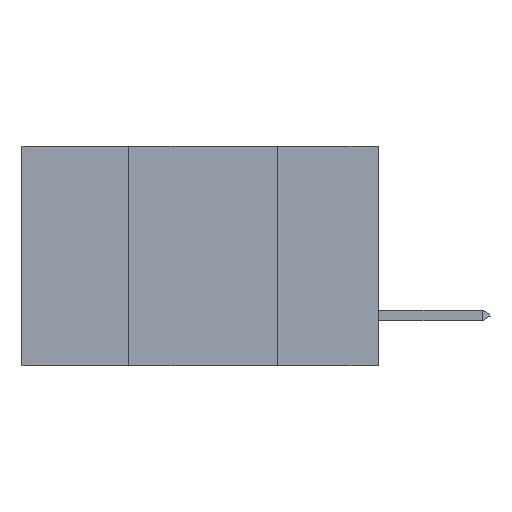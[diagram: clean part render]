
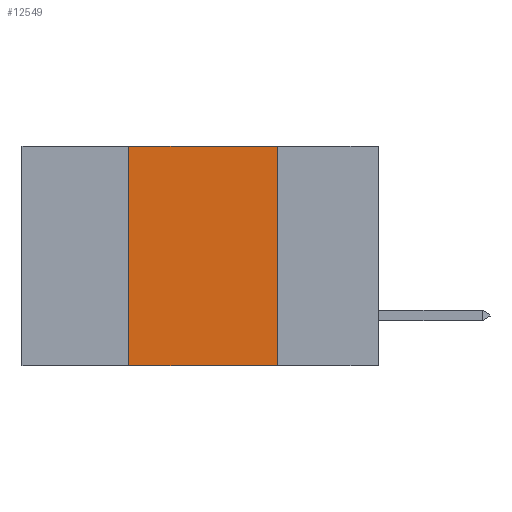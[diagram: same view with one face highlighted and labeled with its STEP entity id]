
A CAD part, left-side view. The second image highlights one B-rep face of the part: STEP entity #12549.
In plain terms, the highlighted planar face has unit normal (-1, 0, 0).
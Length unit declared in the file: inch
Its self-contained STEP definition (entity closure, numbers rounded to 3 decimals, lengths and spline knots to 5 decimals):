
#372 = LINE ( 'NONE', #12339, #6073 ) ;
#637 = EDGE_CURVE ( 'NONE', #7337, #4978, #2503, .T. ) ;
#995 = EDGE_CURVE ( 'NONE', #4978, #8960, #372, .T. ) ;
#1590 = LINE ( 'NONE', #6500, #5011 ) ;
#1611 = CARTESIAN_POINT ( 'NONE',  ( 0., 0.6, 0. ) ) ;
#1785 = DIRECTION ( 'NONE',  ( 0., 0., -1. ) ) ;
#2177 = VERTEX_POINT ( 'NONE', #12095 ) ;
#2503 = LINE ( 'NONE', #1611, #7447 ) ;
#2643 = CARTESIAN_POINT ( 'NONE',  ( 0., 0.6, -0.37 ) ) ;
#2696 = DIRECTION ( 'NONE',  ( 0., -1., 0. ) ) ;
#2707 = VECTOR ( 'NONE', #7983, 39.37008 ) ;
#3459 = EDGE_LOOP ( 'NONE', ( #6336, #8655, #12703, #9341 ) ) ;
#4978 = VERTEX_POINT ( 'NONE', #8935 ) ;
#5011 = VECTOR ( 'NONE', #10710, 39.37008 ) ;
#5422 = EDGE_CURVE ( 'NONE', #2177, #8960, #8772, .T. ) ;
#6073 = VECTOR ( 'NONE', #1785, 39.37008 ) ;
#6336 = ORIENTED_EDGE ( 'NONE', *, *, #995, .F. ) ;
#6500 = CARTESIAN_POINT ( 'NONE',  ( 0., 0.42, 0. ) ) ;
#7302 = DIRECTION ( 'NONE',  ( 1., 0., 0. ) ) ;
#7337 = VERTEX_POINT ( 'NONE', #11039 ) ;
#7447 = VECTOR ( 'NONE', #2696, 39.37008 ) ;
#7983 = DIRECTION ( 'NONE',  ( 0., -1., 0. ) ) ;
#8436 = DIRECTION ( 'NONE',  ( 0., 0., -1. ) ) ;
#8479 = CARTESIAN_POINT ( 'NONE',  ( 0., 0.6, 0. ) ) ;
#8655 = ORIENTED_EDGE ( 'NONE', *, *, #637, .F. ) ;
#8772 = LINE ( 'NONE', #2643, #2707 ) ;
#8935 = CARTESIAN_POINT ( 'NONE',  ( 0., 0.17, 0. ) ) ;
#8960 = VERTEX_POINT ( 'NONE', #12681 ) ;
#9333 = PLANE ( 'NONE',  #11163 ) ;
#9341 = ORIENTED_EDGE ( 'NONE', *, *, #5422, .T. ) ;
#10710 = DIRECTION ( 'NONE',  ( 0., 0., 1. ) ) ;
#11039 = CARTESIAN_POINT ( 'NONE',  ( 0., 0.42, 0. ) ) ;
#11163 = AXIS2_PLACEMENT_3D ( 'NONE', #8479, #7302, #8436 ) ;
#11909 = EDGE_CURVE ( 'NONE', #2177, #7337, #1590, .T. ) ;
#11938 = FACE_OUTER_BOUND ( 'NONE', #3459, .T. ) ;
#12095 = CARTESIAN_POINT ( 'NONE',  ( 0., 0.42, -0.37 ) ) ;
#12339 = CARTESIAN_POINT ( 'NONE',  ( 0., 0.17, 0. ) ) ;
#12549 = ADVANCED_FACE ( 'NONE', ( #11938 ), #9333, .F. ) ;
#12681 = CARTESIAN_POINT ( 'NONE',  ( 0., 0.17, -0.37 ) ) ;
#12703 = ORIENTED_EDGE ( 'NONE', *, *, #11909, .F. ) ;
